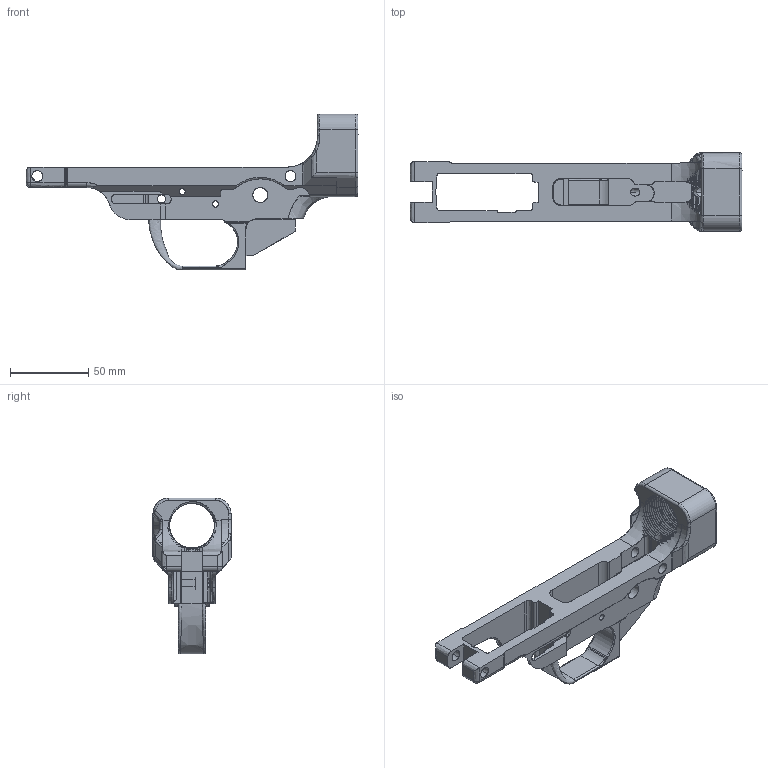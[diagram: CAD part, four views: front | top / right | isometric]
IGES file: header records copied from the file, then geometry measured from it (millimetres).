
Start section: SolidWorks IGES file using analytic representation for surfaces
Global section: file name: Phobos_V1.2.IGS; native system: SolidWorks 2015; preprocessor: SolidWorks 2015; author: WarFairy; date: 150521.090753; units: inch
Bounding box: 212.37 x 50 x 99.72 mm (x, y, z)
Surface area: 49014.8 mm2 (no closed solid volume)
Topology: 0 solids, 0 shells, 475 faces, 5987 edges, 5974 vertices
Faces by surface type: bspline 238, revolution 237
